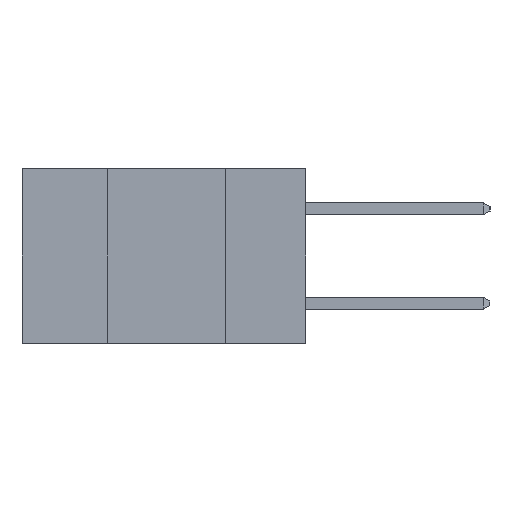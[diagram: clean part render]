
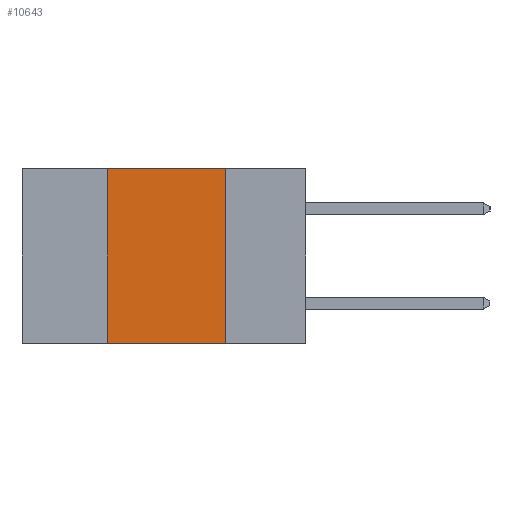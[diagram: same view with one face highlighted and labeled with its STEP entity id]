
A CAD part, left-side view. The second image highlights one B-rep face of the part: STEP entity #10643.
In plain terms, the highlighted planar face has unit normal (-1, 0, 0).
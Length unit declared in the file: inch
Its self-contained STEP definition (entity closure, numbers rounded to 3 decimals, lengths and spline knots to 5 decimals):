
#44 = DIRECTION ( 'NONE',  ( 0., -1., 0. ) ) ;
#54 = VECTOR ( 'NONE', #3146, 39.37008 ) ;
#210 = DIRECTION ( 'NONE',  ( 0., 0., -1. ) ) ;
#862 = CARTESIAN_POINT ( 'NONE',  ( 0., 0.42, -0.37 ) ) ;
#964 = VECTOR ( 'NONE', #6878, 39.37008 ) ;
#977 = FACE_OUTER_BOUND ( 'NONE', #2098, .T. ) ;
#1943 = EDGE_CURVE ( 'NONE', #3330, #4182, #6604, .T. ) ;
#2020 = ORIENTED_EDGE ( 'NONE', *, *, #4277, .F. ) ;
#2098 = EDGE_LOOP ( 'NONE', ( #5194, #2020, #2688, #3704 ) ) ;
#2670 = EDGE_CURVE ( 'NONE', #6951, #11616, #11152, .T. ) ;
#2688 = ORIENTED_EDGE ( 'NONE', *, *, #2670, .F. ) ;
#3146 = DIRECTION ( 'NONE',  ( 0., 0., 1. ) ) ;
#3161 = CARTESIAN_POINT ( 'NONE',  ( 0., 0.42, 0. ) ) ;
#3326 = VECTOR ( 'NONE', #44, 39.37008 ) ;
#3330 = VERTEX_POINT ( 'NONE', #4714 ) ;
#3557 = EDGE_CURVE ( 'NONE', #6951, #4182, #8758, .T. ) ;
#3704 = ORIENTED_EDGE ( 'NONE', *, *, #3557, .T. ) ;
#4182 = VERTEX_POINT ( 'NONE', #12426 ) ;
#4277 = EDGE_CURVE ( 'NONE', #11616, #3330, #8576, .T. ) ;
#4714 = CARTESIAN_POINT ( 'NONE',  ( 0., 0.17, 0. ) ) ;
#4738 = AXIS2_PLACEMENT_3D ( 'NONE', #7569, #6613, #210 ) ;
#5194 = ORIENTED_EDGE ( 'NONE', *, *, #1943, .F. ) ;
#6604 = LINE ( 'NONE', #13206, #964 ) ;
#6613 = DIRECTION ( 'NONE',  ( 1., 0., 0. ) ) ;
#6878 = DIRECTION ( 'NONE',  ( 0., 0., -1. ) ) ;
#6951 = VERTEX_POINT ( 'NONE', #862 ) ;
#7569 = CARTESIAN_POINT ( 'NONE',  ( 0., 0.6, 0. ) ) ;
#8576 = LINE ( 'NONE', #8999, #10952 ) ;
#8758 = LINE ( 'NONE', #10372, #3326 ) ;
#8999 = CARTESIAN_POINT ( 'NONE',  ( 0., 0.6, 0. ) ) ;
#9988 = CARTESIAN_POINT ( 'NONE',  ( 0., 0.42, 0. ) ) ;
#10372 = CARTESIAN_POINT ( 'NONE',  ( 0., 0.6, -0.37 ) ) ;
#10643 = ADVANCED_FACE ( 'NONE', ( #977 ), #12568, .F. ) ;
#10952 = VECTOR ( 'NONE', #12770, 39.37008 ) ;
#11152 = LINE ( 'NONE', #3161, #54 ) ;
#11616 = VERTEX_POINT ( 'NONE', #9988 ) ;
#12426 = CARTESIAN_POINT ( 'NONE',  ( 0., 0.17, -0.37 ) ) ;
#12568 = PLANE ( 'NONE',  #4738 ) ;
#12770 = DIRECTION ( 'NONE',  ( 0., -1., 0. ) ) ;
#13206 = CARTESIAN_POINT ( 'NONE',  ( 0., 0.17, 0. ) ) ;
